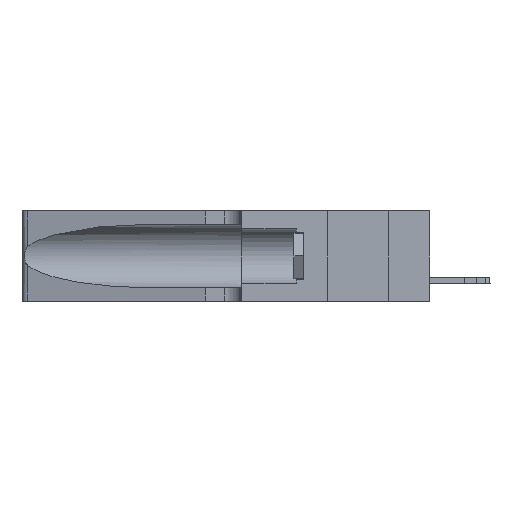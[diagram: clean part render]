
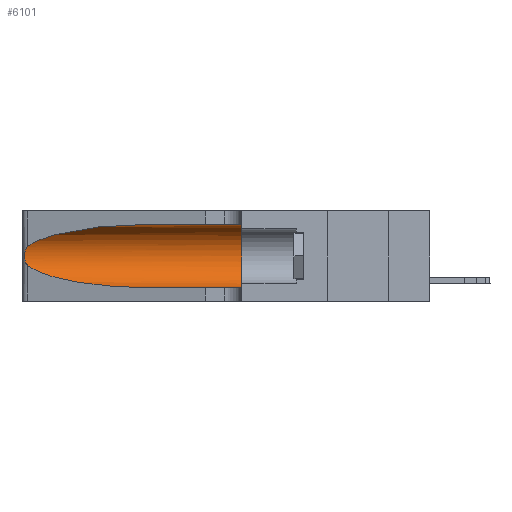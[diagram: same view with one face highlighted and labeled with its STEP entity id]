
A CAD part, left-side view. The second image highlights one B-rep face of the part: STEP entity #6101.
In plain terms, the highlighted cylindrical face has radius 3.308 mm (diameter 6.617 mm), a partial arc.
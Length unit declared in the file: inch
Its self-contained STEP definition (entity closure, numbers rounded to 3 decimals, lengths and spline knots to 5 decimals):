
#952 = B_SPLINE_CURVE_WITH_KNOTS ( 'NONE', 3,
 ( #23753, #5666, #32489, #8435, #5907, #2417, #29353, #29592, #11669, #20638, #38387, #23497, #35777, #26805 ),
 .UNSPECIFIED., .F., .F.,
 ( 4, 2, 2, 2, 2, 2, 4 ),
 ( 0., 0.00027, 0.00053, 0.00107, 0.0016, 0.00187, 0.00214 ),
 .UNSPECIFIED. ) ;
#1140 = VERTEX_POINT ( 'NONE', #30713 ) ;
#1265 = EDGE_LOOP ( 'NONE', ( #21701, #6328, #38538, #33069, #15984, #18469 ) ) ;
#2417 = CARTESIAN_POINT ( 'NONE',  ( 0.26018, 1.23835, 0.19895 ) ) ;
#3302 = DIRECTION ( 'NONE',  ( 0., 1., 0. ) ) ;
#3806 = CARTESIAN_POINT ( 'NONE',  ( 0.25487, 1.22718, 0.14631 ) ) ;
#5666 = CARTESIAN_POINT ( 'NONE',  ( 0.25555, 1.22994, 0.2215 ) ) ;
#5683 = CARTESIAN_POINT ( 'NONE',  ( 0.1305, 1.61858, 0.31525 ) ) ;
#5907 = CARTESIAN_POINT ( 'NONE',  ( 0.25854, 1.2359, 0.20912 ) ) ;
#6101 = ADVANCED_FACE ( 'NONE', ( #9817 ), #32789, .F. ) ;
#6328 = ORIENTED_EDGE ( 'NONE', *, *, #35607, .T. ) ;
#6577 = VERTEX_POINT ( 'NONE', #24608 ) ;
#6802 = CARTESIAN_POINT ( 'NONE',  ( 0.18966, 0.96281, 0.05475 ) ) ;
#7658 = CARTESIAN_POINT ( 'NONE',  ( 0.18966, 0.96281, 0.31525 ) ) ;
#7790 = CARTESIAN_POINT ( 'NONE',  ( 0.25487, 1.22718, 0.22369 ) ) ;
#7988 =( BOUNDED_CURVE ( )  B_SPLINE_CURVE ( 3, ( #3806, #27312, #6802, #27701 ),
 .UNSPECIFIED., .F., .T. ) 
 B_SPLINE_CURVE_WITH_KNOTS ( ( 4, 4 ),
 ( 3.44316, 4.71239 ),
 .UNSPECIFIED. ) 
 CURVE ( )  GEOMETRIC_REPRESENTATION_ITEM ( )  RATIONAL_B_SPLINE_CURVE ( ( 1., 0.87, 0.87, 1. ) ) 
 REPRESENTATION_ITEM ( '' )  );
#8435 = CARTESIAN_POINT ( 'NONE',  ( 0.25787, 1.23484, 0.2124 ) ) ;
#9229 = CIRCLE ( 'NONE', #21714, 0.13025 ) ;
#9817 = FACE_OUTER_BOUND ( 'NONE', #1265, .T. ) ;
#9895 = VERTEX_POINT ( 'NONE', #10230 ) ;
#10230 = CARTESIAN_POINT ( 'NONE',  ( 0.1305, 0.35, 0.05475 ) ) ;
#11669 = CARTESIAN_POINT ( 'NONE',  ( 0.26017, 1.23833, 0.17102 ) ) ;
#12749 = EDGE_CURVE ( 'NONE', #29608, #1140, #13203, .T. ) ;
#13203 =( BOUNDED_CURVE ( )  B_SPLINE_CURVE ( 3, ( #18809, #7658, #19627, #7790 ),
 .UNSPECIFIED., .F., .F. ) 
 B_SPLINE_CURVE_WITH_KNOTS ( ( 4, 4 ),
 ( 1.5708, 2.84003 ),
 .UNSPECIFIED. ) 
 CURVE ( )  GEOMETRIC_REPRESENTATION_ITEM ( )  RATIONAL_B_SPLINE_CURVE ( ( 1., 0.87, 0.87, 1. ) ) 
 REPRESENTATION_ITEM ( '' )  );
#14104 = VERTEX_POINT ( 'NONE', #31433 ) ;
#14926 = EDGE_CURVE ( 'NONE', #22980, #9895, #18513, .T. ) ;
#15129 = VECTOR ( 'NONE', #38412, 39.37008 ) ;
#15300 = DIRECTION ( 'NONE',  ( 0., 0., 1. ) ) ;
#15984 = ORIENTED_EDGE ( 'NONE', *, *, #35204, .F. ) ;
#18469 = ORIENTED_EDGE ( 'NONE', *, *, #28309, .F. ) ;
#18513 = LINE ( 'NONE', #30203, #37346 ) ;
#18809 = CARTESIAN_POINT ( 'NONE',  ( 0.1305, 0.72297, 0.31525 ) ) ;
#19627 = CARTESIAN_POINT ( 'NONE',  ( 0.2373, 1.15595, 0.28018 ) ) ;
#20638 = CARTESIAN_POINT ( 'NONE',  ( 0.25856, 1.23593, 0.16098 ) ) ;
#21701 = ORIENTED_EDGE ( 'NONE', *, *, #12749, .T. ) ;
#21714 = AXIS2_PLACEMENT_3D ( 'NONE', #36153, #3302, #15300 ) ;
#22980 = VERTEX_POINT ( 'NONE', #35186 ) ;
#23497 = CARTESIAN_POINT ( 'NONE',  ( 0.25639, 1.23186, 0.15144 ) ) ;
#23753 = CARTESIAN_POINT ( 'NONE',  ( 0.25487, 1.22718, 0.22369 ) ) ;
#24608 = CARTESIAN_POINT ( 'NONE',  ( 0.1305, 0.35, 0.31525 ) ) ;
#25513 = CARTESIAN_POINT ( 'NONE',  ( 0.1305, 1.61858, 0.185 ) ) ;
#25771 = DIRECTION ( 'NONE',  ( 0., -1., 0. ) ) ;
#26805 = CARTESIAN_POINT ( 'NONE',  ( 0.25487, 1.22718, 0.14631 ) ) ;
#27312 = CARTESIAN_POINT ( 'NONE',  ( 0.2373, 1.15595, 0.08982 ) ) ;
#27701 = CARTESIAN_POINT ( 'NONE',  ( 0.1305, 0.72297, 0.05475 ) ) ;
#28309 = EDGE_CURVE ( 'NONE', #29608, #6577, #29228, .T. ) ;
#29228 = LINE ( 'NONE', #5683, #15129 ) ;
#29353 = CARTESIAN_POINT ( 'NONE',  ( 0.26075, 1.23896, 0.19203 ) ) ;
#29592 = CARTESIAN_POINT ( 'NONE',  ( 0.26075, 1.23896, 0.178 ) ) ;
#29608 = VERTEX_POINT ( 'NONE', #36722 ) ;
#30203 = CARTESIAN_POINT ( 'NONE',  ( 0.1305, 1.61858, 0.05475 ) ) ;
#30713 = CARTESIAN_POINT ( 'NONE',  ( 0.25487, 1.22718, 0.22369 ) ) ;
#31186 = AXIS2_PLACEMENT_3D ( 'NONE', #25513, #25771, #32163 ) ;
#31433 = CARTESIAN_POINT ( 'NONE',  ( 0.25487, 1.22718, 0.14631 ) ) ;
#32163 = DIRECTION ( 'NONE',  ( 0., 0., -1. ) ) ;
#32489 = CARTESIAN_POINT ( 'NONE',  ( 0.25639, 1.23184, 0.21858 ) ) ;
#32789 = CYLINDRICAL_SURFACE ( 'NONE', #31186, 0.13025 ) ;
#33069 = ORIENTED_EDGE ( 'NONE', *, *, #14926, .T. ) ;
#35186 = CARTESIAN_POINT ( 'NONE',  ( 0.1305, 0.72297, 0.05475 ) ) ;
#35204 = EDGE_CURVE ( 'NONE', #6577, #9895, #9229, .T. ) ;
#35607 = EDGE_CURVE ( 'NONE', #1140, #14104, #952, .T. ) ;
#35777 = CARTESIAN_POINT ( 'NONE',  ( 0.25555, 1.22993, 0.14849 ) ) ;
#36153 = CARTESIAN_POINT ( 'NONE',  ( 0.1305, 0.35, 0.185 ) ) ;
#36601 = DIRECTION ( 'NONE',  ( 0., -1., 0. ) ) ;
#36722 = CARTESIAN_POINT ( 'NONE',  ( 0.1305, 0.72297, 0.31525 ) ) ;
#37149 = EDGE_CURVE ( 'NONE', #14104, #22980, #7988, .T. ) ;
#37346 = VECTOR ( 'NONE', #36601, 39.37008 ) ;
#38387 = CARTESIAN_POINT ( 'NONE',  ( 0.25789, 1.23486, 0.15765 ) ) ;
#38412 = DIRECTION ( 'NONE',  ( 0., -1., 0. ) ) ;
#38538 = ORIENTED_EDGE ( 'NONE', *, *, #37149, .T. ) ;
